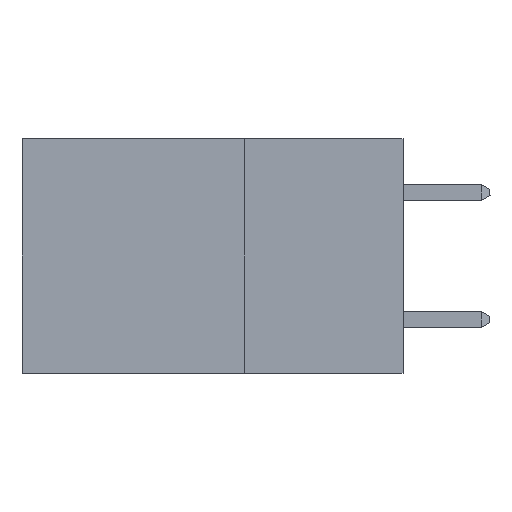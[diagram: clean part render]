
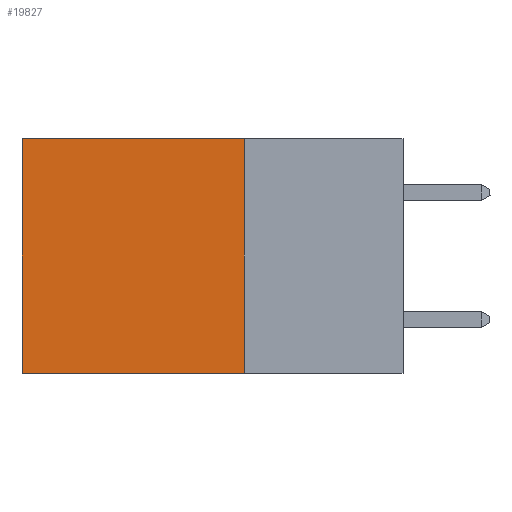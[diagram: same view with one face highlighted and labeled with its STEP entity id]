
A CAD part, left-side view. The second image highlights one B-rep face of the part: STEP entity #19827.
In plain terms, the highlighted planar face has unit normal (-1, 0, 0).
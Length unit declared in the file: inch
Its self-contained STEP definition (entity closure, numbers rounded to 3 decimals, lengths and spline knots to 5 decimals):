
#2073 = CARTESIAN_POINT ( 'NONE',  ( 0.2875, 0.25, -0.37 ) ) ;
#2909 = EDGE_CURVE ( 'NONE', #20065, #33602, #29203, .T. ) ;
#2951 = LINE ( 'NONE', #13333, #37934 ) ;
#5218 = CARTESIAN_POINT ( 'NONE',  ( 0.2875, 0.6, 0. ) ) ;
#5289 = AXIS2_PLACEMENT_3D ( 'NONE', #19042, #31991, #32618 ) ;
#6557 = CARTESIAN_POINT ( 'NONE',  ( 0.2875, 0.25, 0. ) ) ;
#6937 = VERTEX_POINT ( 'NONE', #6557 ) ;
#9955 = DIRECTION ( 'NONE',  ( 0., 0., -1. ) ) ;
#10296 = VECTOR ( 'NONE', #33457, 39.37008 ) ;
#12551 = EDGE_CURVE ( 'NONE', #18238, #33602, #40622, .T. ) ;
#13333 = CARTESIAN_POINT ( 'NONE',  ( 0.2875, 0.25, 0. ) ) ;
#14319 = LINE ( 'NONE', #17295, #14910 ) ;
#14910 = VECTOR ( 'NONE', #27275, 39.37008 ) ;
#16248 = EDGE_LOOP ( 'NONE', ( #21565, #38401, #20180, #38423 ) ) ;
#16267 = PLANE ( 'NONE',  #5289 ) ;
#16675 = CARTESIAN_POINT ( 'NONE',  ( 0.2875, 0.6, 0. ) ) ;
#17295 = CARTESIAN_POINT ( 'NONE',  ( 0.2875, 0.25, 0. ) ) ;
#18238 = VERTEX_POINT ( 'NONE', #2073 ) ;
#19042 = CARTESIAN_POINT ( 'NONE',  ( 0.2875, 0.25, 0. ) ) ;
#19724 = VECTOR ( 'NONE', #35760, 39.37008 ) ;
#19827 = ADVANCED_FACE ( 'NONE', ( #35996 ), #16267, .F. ) ;
#20065 = VERTEX_POINT ( 'NONE', #5218 ) ;
#20180 = ORIENTED_EDGE ( 'NONE', *, *, #37146, .F. ) ;
#21565 = ORIENTED_EDGE ( 'NONE', *, *, #2909, .T. ) ;
#27275 = DIRECTION ( 'NONE',  ( 0., 1., 0. ) ) ;
#29203 = LINE ( 'NONE', #16675, #19724 ) ;
#31991 = DIRECTION ( 'NONE',  ( 1., 0., 0. ) ) ;
#32618 = DIRECTION ( 'NONE',  ( 0., 0., -1. ) ) ;
#33457 = DIRECTION ( 'NONE',  ( 0., 1., 0. ) ) ;
#33602 = VERTEX_POINT ( 'NONE', #35843 ) ;
#34674 = EDGE_CURVE ( 'NONE', #6937, #20065, #14319, .T. ) ;
#35760 = DIRECTION ( 'NONE',  ( 0., 0., -1. ) ) ;
#35843 = CARTESIAN_POINT ( 'NONE',  ( 0.2875, 0.6, -0.37 ) ) ;
#35996 = FACE_OUTER_BOUND ( 'NONE', #16248, .T. ) ;
#36830 = CARTESIAN_POINT ( 'NONE',  ( 0.2875, 0.25, -0.37 ) ) ;
#37146 = EDGE_CURVE ( 'NONE', #6937, #18238, #2951, .T. ) ;
#37934 = VECTOR ( 'NONE', #9955, 39.37008 ) ;
#38401 = ORIENTED_EDGE ( 'NONE', *, *, #12551, .F. ) ;
#38423 = ORIENTED_EDGE ( 'NONE', *, *, #34674, .T. ) ;
#40622 = LINE ( 'NONE', #36830, #10296 ) ;
